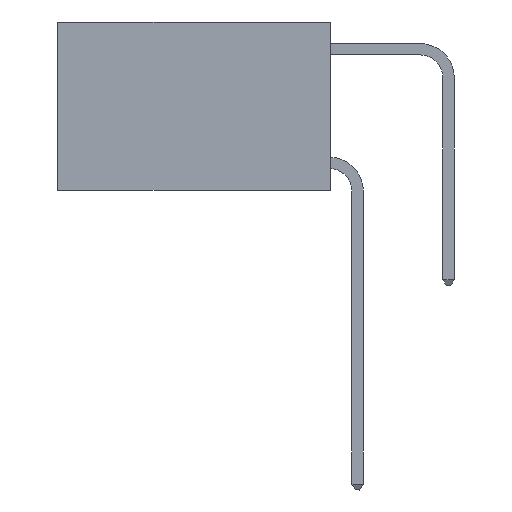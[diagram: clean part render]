
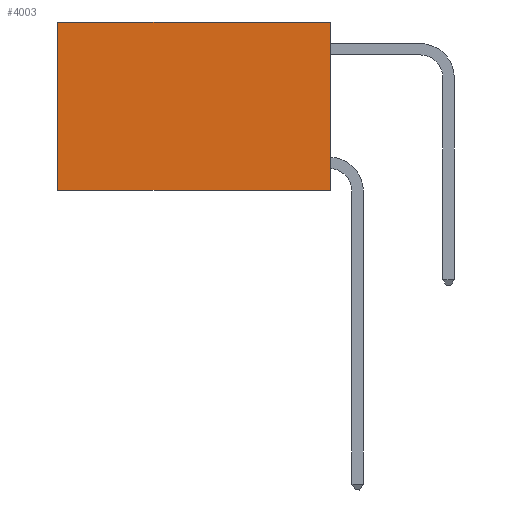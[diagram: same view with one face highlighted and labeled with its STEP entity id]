
A CAD part, left-side view. The second image highlights one B-rep face of the part: STEP entity #4003.
In plain terms, the highlighted planar face has unit normal (-1, 0, 0).
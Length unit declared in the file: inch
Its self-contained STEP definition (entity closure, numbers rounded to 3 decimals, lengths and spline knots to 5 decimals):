
#471 = DIRECTION ( 'NONE',  ( 1., 0., 0. ) ) ;
#704 = EDGE_CURVE ( 'NONE', #2754, #8316, #2198, .T. ) ;
#1767 = CARTESIAN_POINT ( 'NONE',  ( 0.2625, 0.6, -0.37 ) ) ;
#1867 = EDGE_CURVE ( 'NONE', #10018, #5422, #2142, .T. ) ;
#2138 = DIRECTION ( 'NONE',  ( 0., 0., -1. ) ) ;
#2142 = LINE ( 'NONE', #7940, #9464 ) ;
#2198 = LINE ( 'NONE', #2809, #7788 ) ;
#2208 = CARTESIAN_POINT ( 'NONE',  ( 0.2625, 0., 0. ) ) ;
#2250 = EDGE_CURVE ( 'NONE', #5422, #8316, #6307, .T. ) ;
#2754 = VERTEX_POINT ( 'NONE', #5754 ) ;
#2770 = DIRECTION ( 'NONE',  ( 0., 1., 0. ) ) ;
#2809 = CARTESIAN_POINT ( 'NONE',  ( 0.2625, 0., -0.37 ) ) ;
#2934 = CARTESIAN_POINT ( 'NONE',  ( 0.2625, 0.6, 0. ) ) ;
#3171 = EDGE_CURVE ( 'NONE', #10018, #2754, #3555, .T. ) ;
#3523 = FACE_OUTER_BOUND ( 'NONE', #10088, .T. ) ;
#3555 = LINE ( 'NONE', #2208, #5520 ) ;
#3801 = ORIENTED_EDGE ( 'NONE', *, *, #3171, .F. ) ;
#4003 = ADVANCED_FACE ( 'NONE', ( #3523 ), #8479, .F. ) ;
#5422 = VERTEX_POINT ( 'NONE', #5951 ) ;
#5520 = VECTOR ( 'NONE', #6139, 39.37008 ) ;
#5638 = DIRECTION ( 'NONE',  ( 0., 1., 0. ) ) ;
#5754 = CARTESIAN_POINT ( 'NONE',  ( 0.2625, 0., -0.37 ) ) ;
#5951 = CARTESIAN_POINT ( 'NONE',  ( 0.2625, 0.6, 0. ) ) ;
#6139 = DIRECTION ( 'NONE',  ( 0., 0., -1. ) ) ;
#6307 = LINE ( 'NONE', #2934, #8699 ) ;
#6358 = ORIENTED_EDGE ( 'NONE', *, *, #2250, .T. ) ;
#7149 = ORIENTED_EDGE ( 'NONE', *, *, #704, .F. ) ;
#7353 = AXIS2_PLACEMENT_3D ( 'NONE', #10096, #471, #2138 ) ;
#7410 = ORIENTED_EDGE ( 'NONE', *, *, #1867, .T. ) ;
#7659 = CARTESIAN_POINT ( 'NONE',  ( 0.2625, 0., 0. ) ) ;
#7788 = VECTOR ( 'NONE', #2770, 39.37008 ) ;
#7940 = CARTESIAN_POINT ( 'NONE',  ( 0.2625, 0., 0. ) ) ;
#8316 = VERTEX_POINT ( 'NONE', #1767 ) ;
#8459 = DIRECTION ( 'NONE',  ( 0., 0., -1. ) ) ;
#8479 = PLANE ( 'NONE',  #7353 ) ;
#8699 = VECTOR ( 'NONE', #8459, 39.37008 ) ;
#9464 = VECTOR ( 'NONE', #5638, 39.37008 ) ;
#10018 = VERTEX_POINT ( 'NONE', #7659 ) ;
#10088 = EDGE_LOOP ( 'NONE', ( #6358, #7149, #3801, #7410 ) ) ;
#10096 = CARTESIAN_POINT ( 'NONE',  ( 0.2625, 0., 0. ) ) ;
